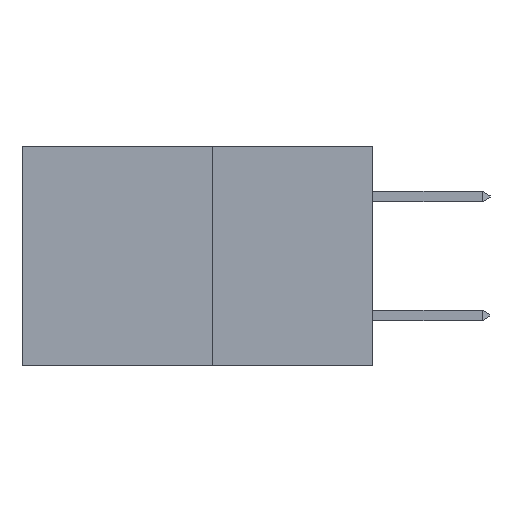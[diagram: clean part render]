
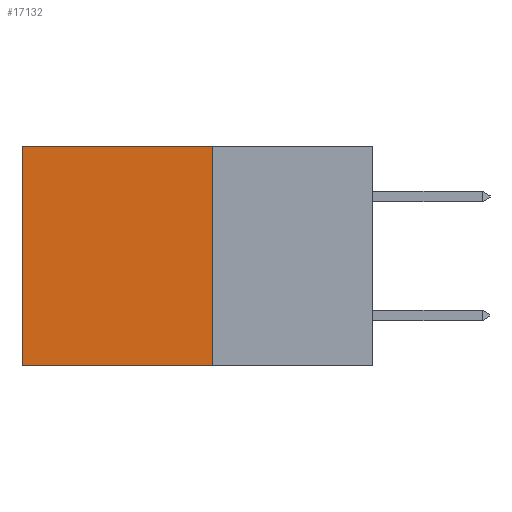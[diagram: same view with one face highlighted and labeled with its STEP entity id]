
A CAD part, left-side view. The second image highlights one B-rep face of the part: STEP entity #17132.
In plain terms, the highlighted planar face has unit normal (-1, 0, 0).
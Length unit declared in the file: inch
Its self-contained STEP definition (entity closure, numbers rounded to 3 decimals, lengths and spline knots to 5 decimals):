
#223 = ORIENTED_EDGE ( 'NONE', *, *, #15346, .F. ) ;
#674 = LINE ( 'NONE', #20334, #9569 ) ;
#843 = DIRECTION ( 'NONE',  ( 0., 1., 0. ) ) ;
#1749 = CARTESIAN_POINT ( 'NONE',  ( 0.277, 0.27, -0.37 ) ) ;
#2260 = EDGE_CURVE ( 'NONE', #12743, #10804, #674, .T. ) ;
#2410 = CARTESIAN_POINT ( 'NONE',  ( 0.277, 0.27, -0.37 ) ) ;
#3248 = EDGE_LOOP ( 'NONE', ( #11449, #16113, #223, #8807 ) ) ;
#3579 = DIRECTION ( 'NONE',  ( 0., 0., -1. ) ) ;
#4196 = LINE ( 'NONE', #1749, #17508 ) ;
#4399 = AXIS2_PLACEMENT_3D ( 'NONE', #13834, #15544, #5129 ) ;
#5129 = DIRECTION ( 'NONE',  ( 0., 0., -1. ) ) ;
#5216 = EDGE_CURVE ( 'NONE', #11701, #10804, #17533, .T. ) ;
#5832 = VERTEX_POINT ( 'NONE', #7315 ) ;
#5889 = CARTESIAN_POINT ( 'NONE',  ( 0.277, 0.59, 0. ) ) ;
#7315 = CARTESIAN_POINT ( 'NONE',  ( 0.277, 0.27, 0. ) ) ;
#7760 = FACE_OUTER_BOUND ( 'NONE', #3248, .T. ) ;
#7835 = VECTOR ( 'NONE', #843, 39.37008 ) ;
#8276 = DIRECTION ( 'NONE',  ( 0., 1., 0. ) ) ;
#8342 = VECTOR ( 'NONE', #13722, 39.37008 ) ;
#8375 = LINE ( 'NONE', #21730, #7835 ) ;
#8807 = ORIENTED_EDGE ( 'NONE', *, *, #20588, .T. ) ;
#9569 = VECTOR ( 'NONE', #8276, 39.37008 ) ;
#10804 = VERTEX_POINT ( 'NONE', #17595 ) ;
#11449 = ORIENTED_EDGE ( 'NONE', *, *, #5216, .T. ) ;
#11701 = VERTEX_POINT ( 'NONE', #5889 ) ;
#12743 = VERTEX_POINT ( 'NONE', #2410 ) ;
#13722 = DIRECTION ( 'NONE',  ( 0., 0., -1. ) ) ;
#13834 = CARTESIAN_POINT ( 'NONE',  ( 0.277, 0.27, -0.37 ) ) ;
#15346 = EDGE_CURVE ( 'NONE', #5832, #12743, #4196, .T. ) ;
#15544 = DIRECTION ( 'NONE',  ( 1., 0., 0. ) ) ;
#16113 = ORIENTED_EDGE ( 'NONE', *, *, #2260, .F. ) ;
#17132 = ADVANCED_FACE ( 'NONE', ( #7760 ), #18925, .F. ) ;
#17508 = VECTOR ( 'NONE', #3579, 39.37008 ) ;
#17533 = LINE ( 'NONE', #18894, #8342 ) ;
#17595 = CARTESIAN_POINT ( 'NONE',  ( 0.277, 0.59, -0.37 ) ) ;
#18894 = CARTESIAN_POINT ( 'NONE',  ( 0.277, 0.59, -0.37 ) ) ;
#18925 = PLANE ( 'NONE',  #4399 ) ;
#20334 = CARTESIAN_POINT ( 'NONE',  ( 0.277, 0.27, -0.37 ) ) ;
#20588 = EDGE_CURVE ( 'NONE', #5832, #11701, #8375, .T. ) ;
#21730 = CARTESIAN_POINT ( 'NONE',  ( 0.277, 0.27, 0. ) ) ;
